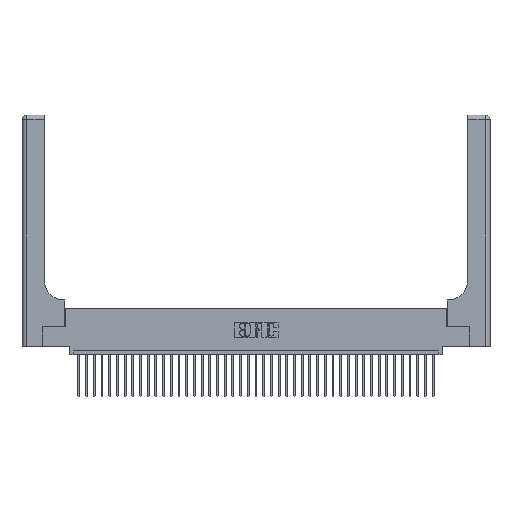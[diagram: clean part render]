
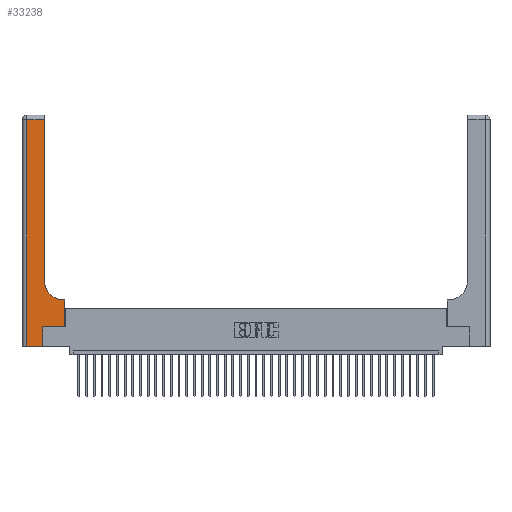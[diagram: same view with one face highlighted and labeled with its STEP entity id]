
A CAD part, top view. The second image highlights one B-rep face of the part: STEP entity #33238.
In plain terms, the highlighted planar face has unit normal (0, 0, 1).
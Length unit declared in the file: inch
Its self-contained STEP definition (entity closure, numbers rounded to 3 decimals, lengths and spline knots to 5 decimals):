
#621 = ORIENTED_EDGE ( 'NONE', *, *, #27599, .T. ) ;
#882 = DIRECTION ( 'NONE',  ( 0., 1., 0. ) ) ;
#995 = DIRECTION ( 'NONE',  ( 1., 0., 0. ) ) ;
#1247 = ORIENTED_EDGE ( 'NONE', *, *, #25313, .T. ) ;
#1257 = VERTEX_POINT ( 'NONE', #13366 ) ;
#1365 = CARTESIAN_POINT ( 'NONE',  ( 0., 0., 0.37 ) ) ;
#1484 = LINE ( 'NONE', #34661, #26144 ) ;
#3731 = VECTOR ( 'NONE', #13002, 39.37008 ) ;
#3958 = CARTESIAN_POINT ( 'NONE',  ( 0.269, 0., 0.37 ) ) ;
#5914 = PLANE ( 'NONE',  #33060 ) ;
#6573 = CARTESIAN_POINT ( 'NONE',  ( 0.2915, 0.85, 0.37 ) ) ;
#6981 = EDGE_CURVE ( 'NONE', #11230, #37957, #10704, .T. ) ;
#9145 = DIRECTION ( 'NONE',  ( -1., 0., 0. ) ) ;
#9622 = VECTOR ( 'NONE', #34878, 39.37008 ) ;
#10365 = ORIENTED_EDGE ( 'NONE', *, *, #34695, .T. ) ;
#10518 = EDGE_LOOP ( 'NONE', ( #18306, #27407, #25187, #621, #1247, #39537, #31825, #10365, #29230 ) ) ;
#10704 = LINE ( 'NONE', #29022, #33924 ) ;
#11230 = VERTEX_POINT ( 'NONE', #13980 ) ;
#11551 = VERTEX_POINT ( 'NONE', #19381 ) ;
#11955 = CARTESIAN_POINT ( 'NONE',  ( 0.06, 2.94, 0.37 ) ) ;
#13002 = DIRECTION ( 'NONE',  ( 0., -1., 0. ) ) ;
#13366 = CARTESIAN_POINT ( 'NONE',  ( 0.5415, 0.6, 0.37 ) ) ;
#13623 = LINE ( 'NONE', #3958, #14086 ) ;
#13980 = CARTESIAN_POINT ( 'NONE',  ( 0.2915, 2.94, 0.37 ) ) ;
#14072 = VERTEX_POINT ( 'NONE', #33607 ) ;
#14086 = VECTOR ( 'NONE', #22352, 39.37008 ) ;
#15784 = VERTEX_POINT ( 'NONE', #17905 ) ;
#17905 = CARTESIAN_POINT ( 'NONE',  ( 0.5585, 0.25, 0.37 ) ) ;
#18005 = LINE ( 'NONE', #27087, #38707 ) ;
#18247 = CIRCLE ( 'NONE', #18766, 0.25 ) ;
#18306 = ORIENTED_EDGE ( 'NONE', *, *, #39530, .T. ) ;
#18477 = VERTEX_POINT ( 'NONE', #24410 ) ;
#18766 = AXIS2_PLACEMENT_3D ( 'NONE', #19314, #38133, #995 ) ;
#18789 = LINE ( 'NONE', #25406, #3731 ) ;
#18906 = VERTEX_POINT ( 'NONE', #20227 ) ;
#19314 = CARTESIAN_POINT ( 'NONE',  ( 0.5415, 0.85, 0.37 ) ) ;
#19381 = CARTESIAN_POINT ( 'NONE',  ( 0.269, 0.25, 0.37 ) ) ;
#20227 = CARTESIAN_POINT ( 'NONE',  ( 0.5585, 0.6, 0.37 ) ) ;
#22352 = DIRECTION ( 'NONE',  ( 0., 1., 0. ) ) ;
#22717 = DIRECTION ( 'NONE',  ( 1., 0., 0. ) ) ;
#23420 = DIRECTION ( 'NONE',  ( 0., 1., 0. ) ) ;
#24170 = DIRECTION ( 'NONE',  ( 0., 0., -1. ) ) ;
#24373 = DIRECTION ( 'NONE',  ( 1., 0., 0. ) ) ;
#24410 = CARTESIAN_POINT ( 'NONE',  ( 0.269, 0., 0.37 ) ) ;
#25187 = ORIENTED_EDGE ( 'NONE', *, *, #29862, .T. ) ;
#25246 = EDGE_CURVE ( 'NONE', #11551, #15784, #18005, .T. ) ;
#25313 = EDGE_CURVE ( 'NONE', #18477, #11551, #13623, .T. ) ;
#25406 = CARTESIAN_POINT ( 'NONE',  ( 0.06, 3., 0.37 ) ) ;
#25678 = FACE_OUTER_BOUND ( 'NONE', #10518, .T. ) ;
#26029 = DIRECTION ( 'NONE',  ( -1., 0., 0. ) ) ;
#26144 = VECTOR ( 'NONE', #882, 39.37008 ) ;
#26196 = VECTOR ( 'NONE', #23420, 39.37008 ) ;
#27087 = CARTESIAN_POINT ( 'NONE',  ( 0.269, 0.25, 0.37 ) ) ;
#27407 = ORIENTED_EDGE ( 'NONE', *, *, #6981, .T. ) ;
#27599 = EDGE_CURVE ( 'NONE', #14072, #18477, #39069, .T. ) ;
#28469 = EDGE_CURVE ( 'NONE', #1257, #30446, #18247, .T. ) ;
#29022 = CARTESIAN_POINT ( 'NONE',  ( 0., 2.94, 0.37 ) ) ;
#29230 = ORIENTED_EDGE ( 'NONE', *, *, #28469, .T. ) ;
#29442 = LINE ( 'NONE', #31227, #9622 ) ;
#29862 = EDGE_CURVE ( 'NONE', #37957, #14072, #18789, .T. ) ;
#30446 = VERTEX_POINT ( 'NONE', #6573 ) ;
#30506 = CARTESIAN_POINT ( 'NONE',  ( 0., 3., 0.37 ) ) ;
#30534 = LINE ( 'NONE', #36107, #26196 ) ;
#31227 = CARTESIAN_POINT ( 'NONE',  ( 0.2915, 0.6, 0.37 ) ) ;
#31825 = ORIENTED_EDGE ( 'NONE', *, *, #39199, .T. ) ;
#33060 = AXIS2_PLACEMENT_3D ( 'NONE', #30506, #24170, #9145 ) ;
#33238 = ADVANCED_FACE ( 'NONE', ( #25678 ), #5914, .F. ) ;
#33607 = CARTESIAN_POINT ( 'NONE',  ( 0.06, 0., 0.37 ) ) ;
#33924 = VECTOR ( 'NONE', #26029, 39.37008 ) ;
#34661 = CARTESIAN_POINT ( 'NONE',  ( 0.5585, 0.25, 0.37 ) ) ;
#34695 = EDGE_CURVE ( 'NONE', #18906, #1257, #29442, .T. ) ;
#34878 = DIRECTION ( 'NONE',  ( -1., 0., 0. ) ) ;
#36107 = CARTESIAN_POINT ( 'NONE',  ( 0.2915, 3., 0.37 ) ) ;
#37135 = VECTOR ( 'NONE', #22717, 39.37008 ) ;
#37957 = VERTEX_POINT ( 'NONE', #11955 ) ;
#38133 = DIRECTION ( 'NONE',  ( 0., 0., -1. ) ) ;
#38707 = VECTOR ( 'NONE', #24373, 39.37008 ) ;
#39069 = LINE ( 'NONE', #1365, #37135 ) ;
#39199 = EDGE_CURVE ( 'NONE', #15784, #18906, #1484, .T. ) ;
#39530 = EDGE_CURVE ( 'NONE', #30446, #11230, #30534, .T. ) ;
#39537 = ORIENTED_EDGE ( 'NONE', *, *, #25246, .T. ) ;
